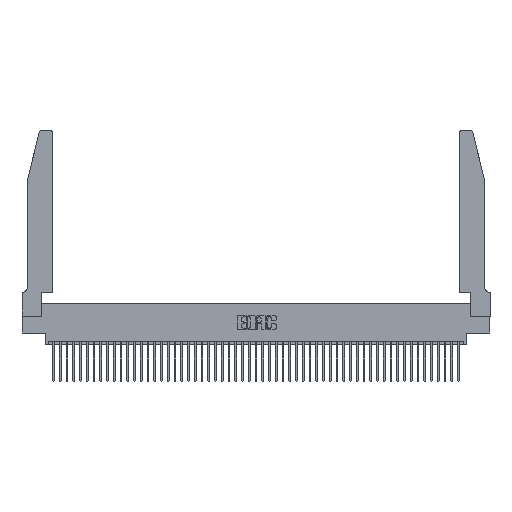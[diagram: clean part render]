
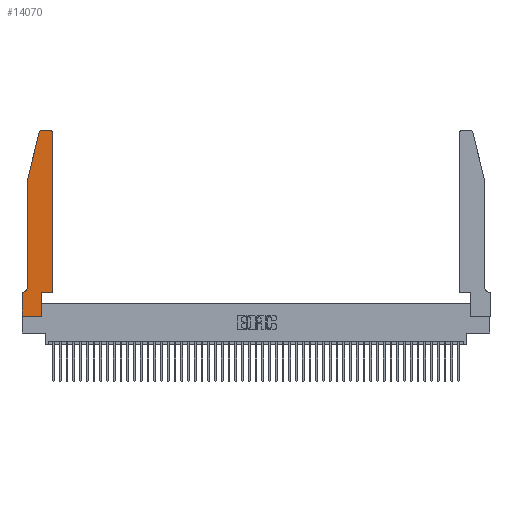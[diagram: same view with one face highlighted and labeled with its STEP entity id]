
A CAD part, top view. The second image highlights one B-rep face of the part: STEP entity #14070.
In plain terms, the highlighted planar face has unit normal (0, 0, 1).
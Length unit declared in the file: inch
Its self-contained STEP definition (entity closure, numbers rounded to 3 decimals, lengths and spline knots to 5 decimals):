
#1045 = LINE ( 'NONE', #46187, #40475 ) ;
#1656 = DIRECTION ( 'NONE',  ( 1., 0., 0. ) ) ;
#2683 = DIRECTION ( 'NONE',  ( 1., 0., 0. ) ) ;
#2734 = VERTEX_POINT ( 'NONE', #21498 ) ;
#3939 = LINE ( 'NONE', #16083, #19811 ) ;
#5426 = LINE ( 'NONE', #34700, #18262 ) ;
#5797 = CARTESIAN_POINT ( 'NONE',  ( 0.4205, 2.72, 0.37 ) ) ;
#5849 = FACE_OUTER_BOUND ( 'NONE', #31182, .T. ) ;
#5870 = DIRECTION ( 'NONE',  ( 0., -1., 0. ) ) ;
#7620 = VERTEX_POINT ( 'NONE', #38421 ) ;
#7625 = VECTOR ( 'NONE', #16028, 39.37008 ) ;
#8855 = CARTESIAN_POINT ( 'NONE',  ( 0.0755, 2., 0.37 ) ) ;
#9004 = VECTOR ( 'NONE', #18411, 39.37008 ) ;
#9463 = CARTESIAN_POINT ( 'NONE',  ( 0., 0., 0.37 ) ) ;
#9744 = LINE ( 'NONE', #8855, #17086 ) ;
#10158 = CARTESIAN_POINT ( 'NONE',  ( 0., 0.35, 0.37 ) ) ;
#11526 = CARTESIAN_POINT ( 'NONE',  ( 0.0755, 0.42, 0.37 ) ) ;
#13643 = VERTEX_POINT ( 'NONE', #22603 ) ;
#14050 = DIRECTION ( 'NONE',  ( 1., 0., 0. ) ) ;
#14070 = ADVANCED_FACE ( 'NONE', ( #5849 ), #33378, .T. ) ;
#14958 = EDGE_CURVE ( 'NONE', #34757, #28498, #27666, .T. ) ;
#15340 = LINE ( 'NONE', #9463, #17811 ) ;
#16028 = DIRECTION ( 'NONE',  ( -1., 0., 0. ) ) ;
#16083 = CARTESIAN_POINT ( 'NONE',  ( 0.0755, 2., 0.37 ) ) ;
#16436 = LINE ( 'NONE', #47795, #20087 ) ;
#16865 = DIRECTION ( 'NONE',  ( 0., -1., 0. ) ) ;
#17070 = CARTESIAN_POINT ( 'NONE',  ( 0.4505, 2.72, 0.37 ) ) ;
#17086 = VECTOR ( 'NONE', #16865, 39.37008 ) ;
#17272 = EDGE_CURVE ( 'NONE', #25325, #7620, #15340, .T. ) ;
#17399 = VERTEX_POINT ( 'NONE', #49074 ) ;
#17771 = ORIENTED_EDGE ( 'NONE', *, *, #44292, .T. ) ;
#17811 = VECTOR ( 'NONE', #5870, 39.37008 ) ;
#18262 = VECTOR ( 'NONE', #42462, 39.37008 ) ;
#18411 = DIRECTION ( 'NONE',  ( 0., 1., 0. ) ) ;
#18541 = EDGE_CURVE ( 'NONE', #17399, #33333, #16436, .T. ) ;
#18995 = CARTESIAN_POINT ( 'NONE',  ( 0.25487, 2.72718, 0.37 ) ) ;
#19459 = EDGE_CURVE ( 'NONE', #33333, #38775, #37524, .T. ) ;
#19811 = VECTOR ( 'NONE', #27977, 39.37008 ) ;
#20087 = VECTOR ( 'NONE', #1656, 39.37008 ) ;
#21070 = DIRECTION ( 'NONE',  ( 1., 0., 0. ) ) ;
#21498 = CARTESIAN_POINT ( 'NONE',  ( 0.0755, 2., 0.37 ) ) ;
#21627 = DIRECTION ( 'NONE',  ( 0., 0., 1. ) ) ;
#22603 = CARTESIAN_POINT ( 'NONE',  ( 0.0055, 0.35, 0.37 ) ) ;
#22826 = AXIS2_PLACEMENT_3D ( 'NONE', #31628, #46535, #23555 ) ;
#23555 = DIRECTION ( 'NONE',  ( -1., 0., 0. ) ) ;
#23958 = ORIENTED_EDGE ( 'NONE', *, *, #34692, .T. ) ;
#25009 = ORIENTED_EDGE ( 'NONE', *, *, #17272, .T. ) ;
#25316 = CIRCLE ( 'NONE', #36383, 0.03 ) ;
#25325 = VERTEX_POINT ( 'NONE', #48397 ) ;
#25362 = CARTESIAN_POINT ( 'NONE',  ( 0.284, 2.75, 0.37 ) ) ;
#26206 = CARTESIAN_POINT ( 'NONE',  ( 0.4505, 0.35, 0.37 ) ) ;
#26676 = ORIENTED_EDGE ( 'NONE', *, *, #28334, .T. ) ;
#27418 = ORIENTED_EDGE ( 'NONE', *, *, #19459, .T. ) ;
#27666 = LINE ( 'NONE', #46344, #7625 ) ;
#27977 = DIRECTION ( 'NONE',  ( -0.239, -0.971, 0. ) ) ;
#28334 = EDGE_CURVE ( 'NONE', #13643, #25325, #1045, .T. ) ;
#28395 = VERTEX_POINT ( 'NONE', #39897 ) ;
#28498 = VERTEX_POINT ( 'NONE', #25362 ) ;
#29083 = LINE ( 'NONE', #37182, #32705 ) ;
#31146 = CARTESIAN_POINT ( 'NONE',  ( 0.4505, 0.35, 0.37 ) ) ;
#31182 = EDGE_LOOP ( 'NONE', ( #31950, #23958, #31368, #17771, #36092, #26676, #25009, #49591, #34842, #45284, #27418, #33031 ) ) ;
#31368 = ORIENTED_EDGE ( 'NONE', *, *, #47526, .T. ) ;
#31628 = CARTESIAN_POINT ( 'NONE',  ( 0.0055, 0.42, 0.37 ) ) ;
#31950 = ORIENTED_EDGE ( 'NONE', *, *, #14958, .T. ) ;
#32705 = VECTOR ( 'NONE', #2683, 39.37008 ) ;
#33031 = ORIENTED_EDGE ( 'NONE', *, *, #36123, .T. ) ;
#33333 = VERTEX_POINT ( 'NONE', #31146 ) ;
#33378 = PLANE ( 'NONE',  #43814 ) ;
#33410 = EDGE_CURVE ( 'NONE', #28395, #17399, #5426, .T. ) ;
#33741 = DIRECTION ( 'NONE',  ( 0., 0., 1. ) ) ;
#33907 = CARTESIAN_POINT ( 'NONE',  ( 0.4205, 2.75, 0.37 ) ) ;
#34272 = EDGE_CURVE ( 'NONE', #7620, #28395, #29083, .T. ) ;
#34692 = EDGE_CURVE ( 'NONE', #28498, #49284, #47799, .T. ) ;
#34700 = CARTESIAN_POINT ( 'NONE',  ( 0.2865, 0.35, 0.37 ) ) ;
#34757 = VERTEX_POINT ( 'NONE', #33907 ) ;
#34842 = ORIENTED_EDGE ( 'NONE', *, *, #33410, .T. ) ;
#34849 = DIRECTION ( 'NONE',  ( -1., 0., 0. ) ) ;
#35032 = AXIS2_PLACEMENT_3D ( 'NONE', #45560, #33741, #21070 ) ;
#36092 = ORIENTED_EDGE ( 'NONE', *, *, #49456, .T. ) ;
#36123 = EDGE_CURVE ( 'NONE', #38775, #34757, #25316, .T. ) ;
#36383 = AXIS2_PLACEMENT_3D ( 'NONE', #5797, #21627, #37362 ) ;
#37182 = CARTESIAN_POINT ( 'NONE',  ( 0., 0., 0.37 ) ) ;
#37299 = DIRECTION ( 'NONE',  ( 0., 0., 1. ) ) ;
#37362 = DIRECTION ( 'NONE',  ( 1., 0., 0. ) ) ;
#37524 = LINE ( 'NONE', #26206, #9004 ) ;
#38421 = CARTESIAN_POINT ( 'NONE',  ( 0., 0., 0.37 ) ) ;
#38775 = VERTEX_POINT ( 'NONE', #17070 ) ;
#39897 = CARTESIAN_POINT ( 'NONE',  ( 0.2865, 0., 0.37 ) ) ;
#40475 = VECTOR ( 'NONE', #34849, 39.37008 ) ;
#42462 = DIRECTION ( 'NONE',  ( 0., 1., 0. ) ) ;
#43814 = AXIS2_PLACEMENT_3D ( 'NONE', #10158, #37299, #14050 ) ;
#44292 = EDGE_CURVE ( 'NONE', #2734, #46487, #9744, .T. ) ;
#44385 = CIRCLE ( 'NONE', #22826, 0.07 ) ;
#45284 = ORIENTED_EDGE ( 'NONE', *, *, #18541, .T. ) ;
#45560 = CARTESIAN_POINT ( 'NONE',  ( 0.284, 2.72, 0.37 ) ) ;
#46187 = CARTESIAN_POINT ( 'NONE',  ( 0.0755, 0.35, 0.37 ) ) ;
#46344 = CARTESIAN_POINT ( 'NONE',  ( 0.2605, 2.75, 0.37 ) ) ;
#46487 = VERTEX_POINT ( 'NONE', #11526 ) ;
#46535 = DIRECTION ( 'NONE',  ( 0., 0., -1. ) ) ;
#47526 = EDGE_CURVE ( 'NONE', #49284, #2734, #3939, .T. ) ;
#47795 = CARTESIAN_POINT ( 'NONE',  ( 0.4505, 0.35, 0.37 ) ) ;
#47799 = CIRCLE ( 'NONE', #35032, 0.03 ) ;
#48397 = CARTESIAN_POINT ( 'NONE',  ( 0., 0.35, 0.37 ) ) ;
#49074 = CARTESIAN_POINT ( 'NONE',  ( 0.2865, 0.35, 0.37 ) ) ;
#49284 = VERTEX_POINT ( 'NONE', #18995 ) ;
#49456 = EDGE_CURVE ( 'NONE', #46487, #13643, #44385, .T. ) ;
#49591 = ORIENTED_EDGE ( 'NONE', *, *, #34272, .T. ) ;
